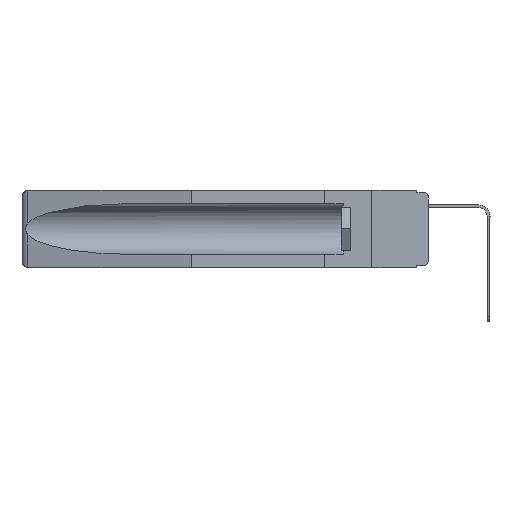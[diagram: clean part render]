
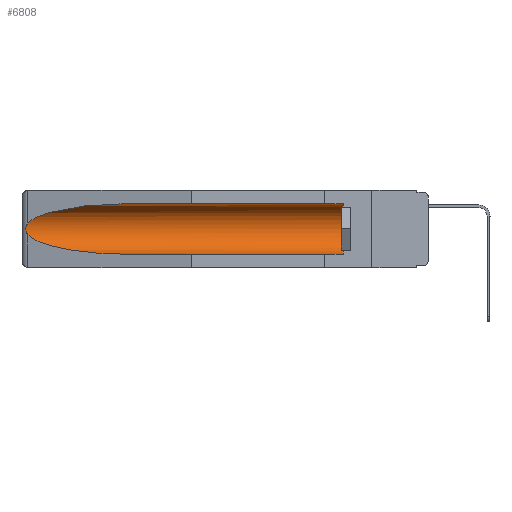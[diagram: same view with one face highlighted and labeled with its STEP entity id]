
A CAD part, left-side view. The second image highlights one B-rep face of the part: STEP entity #6808.
In plain terms, the highlighted cylindrical face has radius 2.857 mm (diameter 5.715 mm), a partial arc.
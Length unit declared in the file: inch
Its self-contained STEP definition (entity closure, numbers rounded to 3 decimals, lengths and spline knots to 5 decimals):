
#1200 = DIRECTION ( 'NONE',  ( 0., 1., 0. ) ) ;
#1216 = ORIENTED_EDGE ( 'NONE', *, *, #10342, .T. ) ;
#1223 = CARTESIAN_POINT ( 'NONE',  ( 0.25451, 1.48313, -0.09465 ) ) ;
#1412 = EDGE_CURVE ( 'NONE', #10580, #9571, #10296, .T. ) ;
#1792 = EDGE_LOOP ( 'NONE', ( #1893, #17574, #1216, #7019, #10381, #6227 ) ) ;
#1893 = ORIENTED_EDGE ( 'NONE', *, *, #20227, .T. ) ;
#1931 = CARTESIAN_POINT ( 'NONE',  ( 0.2673, 1.5327, -0.16383 ) ) ;
#2034 = DIRECTION ( 'NONE',  ( 0., 1., 0. ) ) ;
#2260 = VERTEX_POINT ( 'NONE', #14794 ) ;
#2267 = VERTEX_POINT ( 'NONE', #7510 ) ;
#2642 = CARTESIAN_POINT ( 'NONE',  ( 0.155, 0.126, -0.284 ) ) ;
#3650 = EDGE_CURVE ( 'NONE', #15352, #2260, #18364, .T. ) ;
#4136 = VERTEX_POINT ( 'NONE', #20495 ) ;
#5156 = CARTESIAN_POINT ( 'NONE',  ( 0.25451, 1.48313, -0.24835 ) ) ;
#5290 = CARTESIAN_POINT ( 'NONE',  ( 0.26654, 1.53092, -0.15636 ) ) ;
#5444 = CARTESIAN_POINT ( 'NONE',  ( 0.26597, 1.5296, -0.19026 ) ) ;
#6227 = ORIENTED_EDGE ( 'NONE', *, *, #17044, .T. ) ;
#6421 = CARTESIAN_POINT ( 'NONE',  ( 0.155, -0.30754, -0.284 ) ) ;
#6805 = LINE ( 'NONE', #17528, #17448 ) ;
#6808 = ADVANCED_FACE ( 'NONE', ( #20457 ), #9575, .F. ) ;
#7019 = ORIENTED_EDGE ( 'NONE', *, *, #13669, .F. ) ;
#7236 = CARTESIAN_POINT ( 'NONE',  ( 0.21114, 1.30732, -0.284 ) ) ;
#7510 = CARTESIAN_POINT ( 'NONE',  ( 0.155, 1.07973, -0.284 ) ) ;
#8568 =( BOUNDED_CURVE ( )  B_SPLINE_CURVE ( 3, ( #19131, #5156, #7236, #10683 ),
 .UNSPECIFIED., .F., .F. ) 
 B_SPLINE_CURVE_WITH_KNOTS ( ( 4, 4 ),
 ( 0.1948, 1.5708 ),
 .UNSPECIFIED. ) 
 CURVE ( )  GEOMETRIC_REPRESENTATION_ITEM ( )  RATIONAL_B_SPLINE_CURVE ( ( 1., 0.848, 0.848, 1. ) ) 
 REPRESENTATION_ITEM ( '' )  );
#8804 = DIRECTION ( 'NONE',  ( 0., 0., 1. ) ) ;
#9571 = VERTEX_POINT ( 'NONE', #12554 ) ;
#9575 = CYLINDRICAL_SURFACE ( 'NONE', #19567, 0.1125 ) ;
#10296 = B_SPLINE_CURVE_WITH_KNOTS ( 'NONE', 3,
 ( #10666, #12537, #5290, #1931, #14185, #21287, #17851, #10583, #5444, #12380 ),
 .UNSPECIFIED., .F., .F.,
 ( 4, 2, 2, 2, 4 ),
 ( 0., 0.00029, 0.00058, 0.00087, 0.00117 ),
 .UNSPECIFIED. ) ;
#10342 = EDGE_CURVE ( 'NONE', #9571, #2267, #8568, .T. ) ;
#10350 = DIRECTION ( 'NONE',  ( 0., 1., 0. ) ) ;
#10381 = ORIENTED_EDGE ( 'NONE', *, *, #3650, .T. ) ;
#10580 = VERTEX_POINT ( 'NONE', #22101 ) ;
#10583 = CARTESIAN_POINT ( 'NONE',  ( 0.26655, 1.53094, -0.18657 ) ) ;
#10666 = CARTESIAN_POINT ( 'NONE',  ( 0.26537, 1.52718, -0.14972 ) ) ;
#10683 = CARTESIAN_POINT ( 'NONE',  ( 0.155, 1.07973, -0.284 ) ) ;
#11835 = CARTESIAN_POINT ( 'NONE',  ( 0.26537, 1.52718, -0.14972 ) ) ;
#12380 = CARTESIAN_POINT ( 'NONE',  ( 0.26537, 1.52718, -0.19328 ) ) ;
#12537 = CARTESIAN_POINT ( 'NONE',  ( 0.26597, 1.52961, -0.15275 ) ) ;
#12554 = CARTESIAN_POINT ( 'NONE',  ( 0.26537, 1.52718, -0.19328 ) ) ;
#13483 = DIRECTION ( 'NONE',  ( 0., -1., 0. ) ) ;
#13669 = EDGE_CURVE ( 'NONE', #15352, #2267, #22678, .T. ) ;
#14185 = CARTESIAN_POINT ( 'NONE',  ( 0.2675, 1.53308, -0.16763 ) ) ;
#14794 = CARTESIAN_POINT ( 'NONE',  ( 0.155, 0.126, -0.059 ) ) ;
#15352 = VERTEX_POINT ( 'NONE', #2642 ) ;
#15539 = CARTESIAN_POINT ( 'NONE',  ( 0.21114, 1.30732, -0.059 ) ) ;
#15617 = CARTESIAN_POINT ( 'NONE',  ( 0.155, 1.07973, -0.059 ) ) ;
#16334 = CARTESIAN_POINT ( 'NONE',  ( 0.155, -0.30754, -0.1715 ) ) ;
#17044 = EDGE_CURVE ( 'NONE', #2260, #4136, #6805, .T. ) ;
#17448 = VECTOR ( 'NONE', #10350, 39.37008 ) ;
#17528 = CARTESIAN_POINT ( 'NONE',  ( 0.155, -0.30754, -0.059 ) ) ;
#17574 = ORIENTED_EDGE ( 'NONE', *, *, #1412, .T. ) ;
#17851 = CARTESIAN_POINT ( 'NONE',  ( 0.2673, 1.53269, -0.17917 ) ) ;
#18364 = CIRCLE ( 'NONE', #19984, 0.1125 ) ;
#18598 =( BOUNDED_CURVE ( )  B_SPLINE_CURVE ( 3, ( #15617, #15539, #1223, #11835 ),
 .UNSPECIFIED., .F., .F. ) 
 B_SPLINE_CURVE_WITH_KNOTS ( ( 4, 4 ),
 ( 4.71239, 6.08839 ),
 .UNSPECIFIED. ) 
 CURVE ( )  GEOMETRIC_REPRESENTATION_ITEM ( )  RATIONAL_B_SPLINE_CURVE ( ( 1., 0.848, 0.848, 1. ) ) 
 REPRESENTATION_ITEM ( '' )  );
#19028 = VECTOR ( 'NONE', #1200, 39.37008 ) ;
#19131 = CARTESIAN_POINT ( 'NONE',  ( 0.26537, 1.52718, -0.19328 ) ) ;
#19345 = CARTESIAN_POINT ( 'NONE',  ( 0.155, 0.126, -0.1715 ) ) ;
#19567 = AXIS2_PLACEMENT_3D ( 'NONE', #16334, #2034, #21712 ) ;
#19984 = AXIS2_PLACEMENT_3D ( 'NONE', #19345, #13483, #8804 ) ;
#20227 = EDGE_CURVE ( 'NONE', #4136, #10580, #18598, .T. ) ;
#20457 = FACE_OUTER_BOUND ( 'NONE', #1792, .T. ) ;
#20495 = CARTESIAN_POINT ( 'NONE',  ( 0.155, 1.07973, -0.059 ) ) ;
#21287 = CARTESIAN_POINT ( 'NONE',  ( 0.2675, 1.53308, -0.17534 ) ) ;
#21712 = DIRECTION ( 'NONE',  ( 0., 0., 1. ) ) ;
#22101 = CARTESIAN_POINT ( 'NONE',  ( 0.26537, 1.52718, -0.14972 ) ) ;
#22678 = LINE ( 'NONE', #6421, #19028 ) ;
